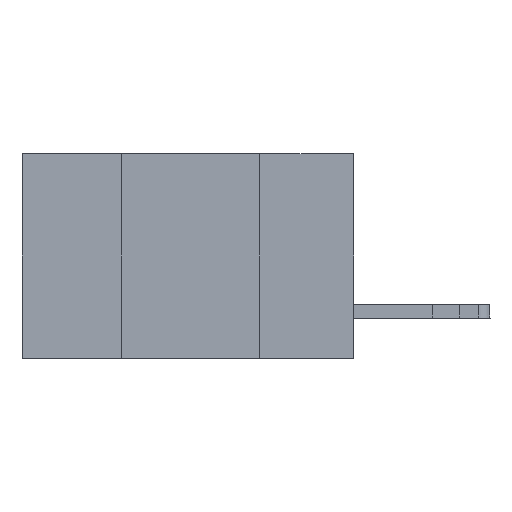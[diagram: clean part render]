
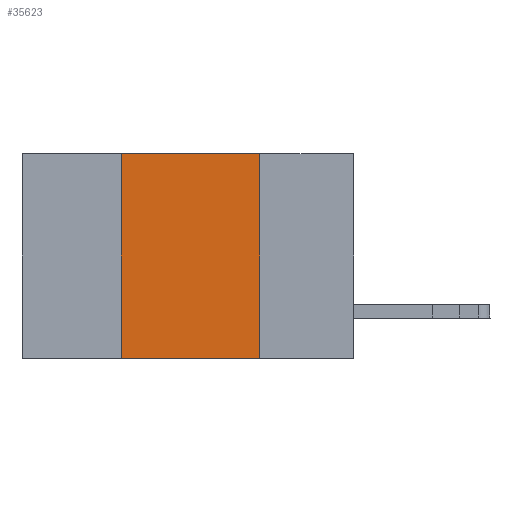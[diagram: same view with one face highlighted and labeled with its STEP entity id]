
A CAD part, left-side view. The second image highlights one B-rep face of the part: STEP entity #35623.
In plain terms, the highlighted planar face has unit normal (-1, 0, 0).
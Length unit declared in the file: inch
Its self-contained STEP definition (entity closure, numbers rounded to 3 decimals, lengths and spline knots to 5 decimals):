
#600 = AXIS2_PLACEMENT_3D ( 'NONE', #8177, #8054, #39322 ) ;
#2018 = VECTOR ( 'NONE', #37844, 39.37008 ) ;
#2164 = DIRECTION ( 'NONE',  ( 0., -1., 0. ) ) ;
#2295 = CARTESIAN_POINT ( 'NONE',  ( 0., 0.42, 0. ) ) ;
#2582 = VECTOR ( 'NONE', #22412, 39.37008 ) ;
#4362 = EDGE_CURVE ( 'NONE', #34972, #14221, #5313, .T. ) ;
#5313 = LINE ( 'NONE', #27210, #34938 ) ;
#5467 = VECTOR ( 'NONE', #2164, 39.37008 ) ;
#5488 = LINE ( 'NONE', #25401, #2582 ) ;
#8054 = DIRECTION ( 'NONE',  ( 1., 0., 0. ) ) ;
#8177 = CARTESIAN_POINT ( 'NONE',  ( 0., 0.6, 0. ) ) ;
#12727 = LINE ( 'NONE', #20637, #5467 ) ;
#13052 = CARTESIAN_POINT ( 'NONE',  ( 0., 0.17, -0.37 ) ) ;
#14221 = VERTEX_POINT ( 'NONE', #2295 ) ;
#14251 = EDGE_CURVE ( 'NONE', #34972, #24556, #24384, .T. ) ;
#16851 = ORIENTED_EDGE ( 'NONE', *, *, #4362, .F. ) ;
#20637 = CARTESIAN_POINT ( 'NONE',  ( 0., 0.6, 0. ) ) ;
#21482 = ORIENTED_EDGE ( 'NONE', *, *, #14251, .T. ) ;
#22412 = DIRECTION ( 'NONE',  ( 0., 0., -1. ) ) ;
#23689 = EDGE_CURVE ( 'NONE', #14221, #39897, #12727, .T. ) ;
#23855 = EDGE_LOOP ( 'NONE', ( #26097, #24417, #16851, #21482 ) ) ;
#24384 = LINE ( 'NONE', #33966, #2018 ) ;
#24417 = ORIENTED_EDGE ( 'NONE', *, *, #23689, .F. ) ;
#24556 = VERTEX_POINT ( 'NONE', #13052 ) ;
#25401 = CARTESIAN_POINT ( 'NONE',  ( 0., 0.17, 0. ) ) ;
#26097 = ORIENTED_EDGE ( 'NONE', *, *, #38325, .F. ) ;
#26150 = CARTESIAN_POINT ( 'NONE',  ( 0., 0.17, 0. ) ) ;
#26694 = PLANE ( 'NONE',  #600 ) ;
#27210 = CARTESIAN_POINT ( 'NONE',  ( 0., 0.42, 0. ) ) ;
#33820 = CARTESIAN_POINT ( 'NONE',  ( 0., 0.42, -0.37 ) ) ;
#33966 = CARTESIAN_POINT ( 'NONE',  ( 0., 0.6, -0.37 ) ) ;
#34938 = VECTOR ( 'NONE', #39569, 39.37008 ) ;
#34972 = VERTEX_POINT ( 'NONE', #33820 ) ;
#35277 = FACE_OUTER_BOUND ( 'NONE', #23855, .T. ) ;
#35623 = ADVANCED_FACE ( 'NONE', ( #35277 ), #26694, .F. ) ;
#37844 = DIRECTION ( 'NONE',  ( 0., -1., 0. ) ) ;
#38325 = EDGE_CURVE ( 'NONE', #39897, #24556, #5488, .T. ) ;
#39322 = DIRECTION ( 'NONE',  ( 0., 0., -1. ) ) ;
#39569 = DIRECTION ( 'NONE',  ( 0., 0., 1. ) ) ;
#39897 = VERTEX_POINT ( 'NONE', #26150 ) ;
